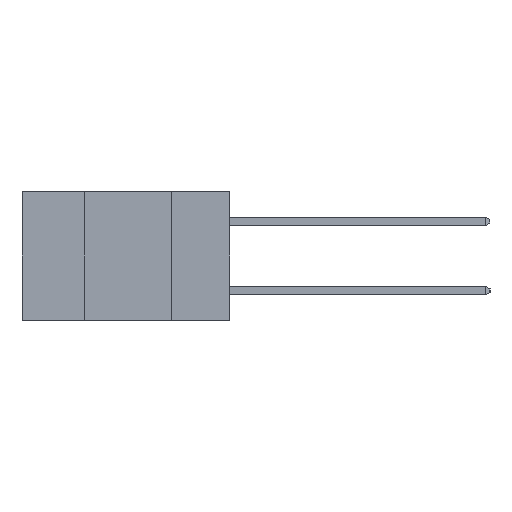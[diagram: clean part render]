
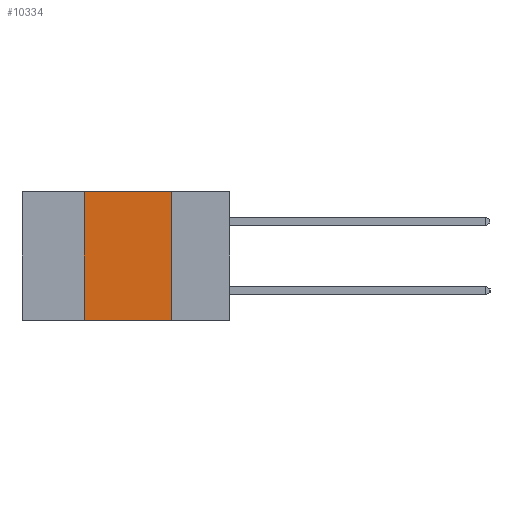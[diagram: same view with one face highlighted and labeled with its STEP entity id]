
A CAD part, left-side view. The second image highlights one B-rep face of the part: STEP entity #10334.
In plain terms, the highlighted planar face has unit normal (-1, 0, 0).
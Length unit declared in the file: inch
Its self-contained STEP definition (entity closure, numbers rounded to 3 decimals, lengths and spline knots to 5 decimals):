
#127 = EDGE_CURVE ( 'NONE', #8812, #9836, #8732, .T. ) ;
#931 = EDGE_LOOP ( 'NONE', ( #5401, #6563, #10053, #10463 ) ) ;
#1859 = DIRECTION ( 'NONE',  ( 0., -1., 0. ) ) ;
#1902 = CARTESIAN_POINT ( 'NONE',  ( 0., 0.6, 0. ) ) ;
#1937 = VERTEX_POINT ( 'NONE', #2723 ) ;
#2463 = DIRECTION ( 'NONE',  ( 0., 0., 1. ) ) ;
#2686 = CARTESIAN_POINT ( 'NONE',  ( 0., 0.42, -0.37 ) ) ;
#2723 = CARTESIAN_POINT ( 'NONE',  ( 0., 0.42, 0. ) ) ;
#2805 = EDGE_CURVE ( 'NONE', #8812, #1937, #15267, .T. ) ;
#2862 = LINE ( 'NONE', #8595, #5875 ) ;
#3672 = EDGE_CURVE ( 'NONE', #1937, #4867, #12429, .T. ) ;
#4668 = CARTESIAN_POINT ( 'NONE',  ( 0., 0.17, 0. ) ) ;
#4867 = VERTEX_POINT ( 'NONE', #4668 ) ;
#5387 = EDGE_CURVE ( 'NONE', #4867, #9836, #2862, .T. ) ;
#5401 = ORIENTED_EDGE ( 'NONE', *, *, #5387, .F. ) ;
#5875 = VECTOR ( 'NONE', #8744, 39.37008 ) ;
#6563 = ORIENTED_EDGE ( 'NONE', *, *, #3672, .F. ) ;
#8595 = CARTESIAN_POINT ( 'NONE',  ( 0., 0.17, -0.37 ) ) ;
#8732 = LINE ( 'NONE', #12776, #11776 ) ;
#8744 = DIRECTION ( 'NONE',  ( 0., 0., -1. ) ) ;
#8812 = VERTEX_POINT ( 'NONE', #9544 ) ;
#8914 = DIRECTION ( 'NONE',  ( 0., 0., -1. ) ) ;
#8933 = DIRECTION ( 'NONE',  ( 1., 0., 0. ) ) ;
#8947 = PLANE ( 'NONE',  #11625 ) ;
#8950 = CARTESIAN_POINT ( 'NONE',  ( 0., 0.6, 0. ) ) ;
#9410 = VECTOR ( 'NONE', #1859, 39.37008 ) ;
#9544 = CARTESIAN_POINT ( 'NONE',  ( 0., 0.42, -0.37 ) ) ;
#9836 = VERTEX_POINT ( 'NONE', #12372 ) ;
#10053 = ORIENTED_EDGE ( 'NONE', *, *, #2805, .F. ) ;
#10334 = ADVANCED_FACE ( 'NONE', ( #12778 ), #8947, .F. ) ;
#10463 = ORIENTED_EDGE ( 'NONE', *, *, #127, .T. ) ;
#11056 = VECTOR ( 'NONE', #2463, 39.37008 ) ;
#11625 = AXIS2_PLACEMENT_3D ( 'NONE', #8950, #8933, #8914 ) ;
#11776 = VECTOR ( 'NONE', #14034, 39.37008 ) ;
#12372 = CARTESIAN_POINT ( 'NONE',  ( 0., 0.17, -0.37 ) ) ;
#12429 = LINE ( 'NONE', #1902, #9410 ) ;
#12776 = CARTESIAN_POINT ( 'NONE',  ( 0., 0.6, -0.37 ) ) ;
#12778 = FACE_OUTER_BOUND ( 'NONE', #931, .T. ) ;
#14034 = DIRECTION ( 'NONE',  ( 0., -1., 0. ) ) ;
#15267 = LINE ( 'NONE', #2686, #11056 ) ;
